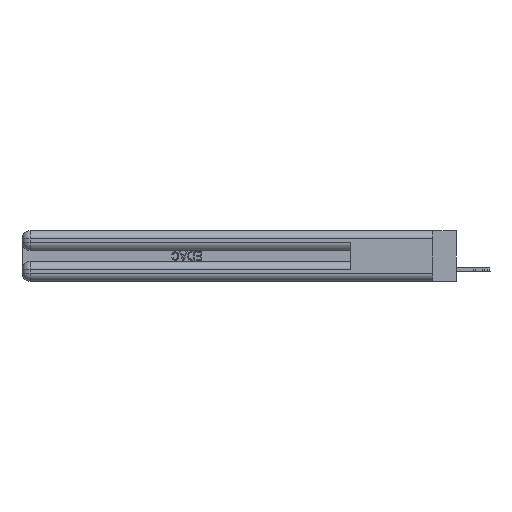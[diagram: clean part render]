
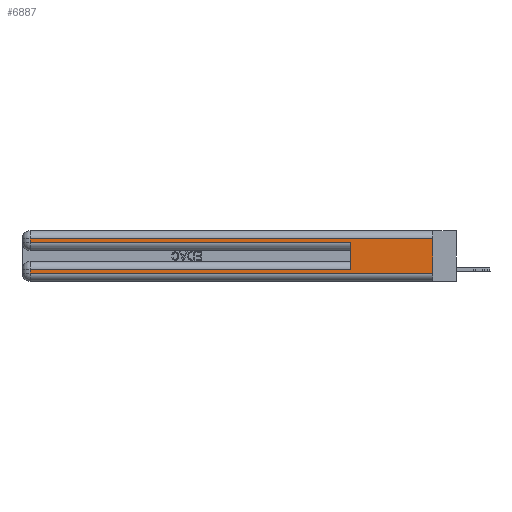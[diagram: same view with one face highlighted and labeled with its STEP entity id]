
A CAD part, left-side view. The second image highlights one B-rep face of the part: STEP entity #6887.
In plain terms, the highlighted planar face has unit normal (-1, 0, 0).
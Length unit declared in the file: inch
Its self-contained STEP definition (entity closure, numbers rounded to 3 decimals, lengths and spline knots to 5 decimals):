
#11 = CARTESIAN_POINT ( 'NONE',  ( 0., 0.6, 0.085 ) ) ;
#498 = VERTEX_POINT ( 'NONE', #2734 ) ;
#561 = LINE ( 'NONE', #31808, #43504 ) ;
#654 = VECTOR ( 'NONE', #34035, 39.37008 ) ;
#1411 = VERTEX_POINT ( 'NONE', #39035 ) ;
#1897 = CARTESIAN_POINT ( 'NONE',  ( 0., 0.6, 0.145 ) ) ;
#2085 = ORIENTED_EDGE ( 'NONE', *, *, #21250, .T. ) ;
#2146 = CARTESIAN_POINT ( 'NONE',  ( 0., 0., 0.06 ) ) ;
#2382 = EDGE_CURVE ( 'NONE', #1411, #4614, #21371, .T. ) ;
#2734 = CARTESIAN_POINT ( 'NONE',  ( 0., 0., 0.31 ) ) ;
#3222 = DIRECTION ( 'NONE',  ( 0., 0., -1. ) ) ;
#4614 = VERTEX_POINT ( 'NONE', #2146 ) ;
#5130 = CARTESIAN_POINT ( 'NONE',  ( 0., 0., 0.31 ) ) ;
#5215 = VERTEX_POINT ( 'NONE', #11 ) ;
#5454 = DIRECTION ( 'NONE',  ( 0., -1., 0. ) ) ;
#5567 = EDGE_CURVE ( 'NONE', #498, #4614, #10279, .T. ) ;
#5962 = CARTESIAN_POINT ( 'NONE',  ( 0., 0., 0.37 ) ) ;
#6195 = DIRECTION ( 'NONE',  ( 0., 0., -1. ) ) ;
#6257 = CARTESIAN_POINT ( 'NONE',  ( 0., 2.94, 0.31 ) ) ;
#6773 = ORIENTED_EDGE ( 'NONE', *, *, #25665, .T. ) ;
#6783 = VECTOR ( 'NONE', #5454, 39.37008 ) ;
#6887 = ADVANCED_FACE ( 'NONE', ( #19415 ), #13083, .F. ) ;
#7236 = CARTESIAN_POINT ( 'NONE',  ( 0., 2.94, 0.37 ) ) ;
#9448 = VECTOR ( 'NONE', #37033, 39.37008 ) ;
#9845 = VERTEX_POINT ( 'NONE', #15299 ) ;
#10125 = VERTEX_POINT ( 'NONE', #23908 ) ;
#10279 = LINE ( 'NONE', #17051, #654 ) ;
#10758 = ORIENTED_EDGE ( 'NONE', *, *, #46274, .T. ) ;
#12896 = CARTESIAN_POINT ( 'NONE',  ( 0., 0., 0.285 ) ) ;
#13076 = DIRECTION ( 'NONE',  ( 0., 0., 1. ) ) ;
#13083 = PLANE ( 'NONE',  #28054 ) ;
#13806 = ORIENTED_EDGE ( 'NONE', *, *, #2382, .T. ) ;
#15299 = CARTESIAN_POINT ( 'NONE',  ( 0., 2.94, 0.085 ) ) ;
#17051 = CARTESIAN_POINT ( 'NONE',  ( 0., 0., 0.37 ) ) ;
#17056 = DIRECTION ( 'NONE',  ( 0., 0., -1. ) ) ;
#17490 = DIRECTION ( 'NONE',  ( 0., 1., 0. ) ) ;
#18004 = ORIENTED_EDGE ( 'NONE', *, *, #33698, .F. ) ;
#19415 = FACE_OUTER_BOUND ( 'NONE', #30570, .T. ) ;
#19613 = VECTOR ( 'NONE', #13076, 39.37008 ) ;
#20991 = VECTOR ( 'NONE', #17490, 39.37008 ) ;
#21250 = EDGE_CURVE ( 'NONE', #5215, #9845, #46392, .T. ) ;
#21371 = LINE ( 'NONE', #37505, #9448 ) ;
#21771 = ORIENTED_EDGE ( 'NONE', *, *, #5567, .F. ) ;
#22453 = VECTOR ( 'NONE', #34040, 39.37008 ) ;
#23908 = CARTESIAN_POINT ( 'NONE',  ( 0., 2.94, 0.285 ) ) ;
#24373 = LINE ( 'NONE', #12896, #6783 ) ;
#25665 = EDGE_CURVE ( 'NONE', #30030, #10125, #561, .T. ) ;
#27537 = LINE ( 'NONE', #1897, #19613 ) ;
#28054 = AXIS2_PLACEMENT_3D ( 'NONE', #5962, #45623, #17056 ) ;
#29434 = VECTOR ( 'NONE', #3222, 39.37008 ) ;
#29924 = CARTESIAN_POINT ( 'NONE',  ( 0., 0.6, 0.285 ) ) ;
#30030 = VERTEX_POINT ( 'NONE', #6257 ) ;
#30570 = EDGE_LOOP ( 'NONE', ( #21771, #36864, #6773, #10758, #18004, #2085, #33802, #13806 ) ) ;
#31808 = CARTESIAN_POINT ( 'NONE',  ( 0., 2.94, 0.37 ) ) ;
#33698 = EDGE_CURVE ( 'NONE', #5215, #41396, #27537, .T. ) ;
#33802 = ORIENTED_EDGE ( 'NONE', *, *, #45904, .T. ) ;
#34035 = DIRECTION ( 'NONE',  ( 0., 0., -1. ) ) ;
#34040 = DIRECTION ( 'NONE',  ( 0., 1., 0. ) ) ;
#36864 = ORIENTED_EDGE ( 'NONE', *, *, #41401, .T. ) ;
#37033 = DIRECTION ( 'NONE',  ( 0., -1., 0. ) ) ;
#37505 = CARTESIAN_POINT ( 'NONE',  ( 0., 0., 0.06 ) ) ;
#38640 = CARTESIAN_POINT ( 'NONE',  ( 0., 0., 0.085 ) ) ;
#39035 = CARTESIAN_POINT ( 'NONE',  ( 0., 2.94, 0.06 ) ) ;
#40505 = LINE ( 'NONE', #5130, #22453 ) ;
#41396 = VERTEX_POINT ( 'NONE', #29924 ) ;
#41401 = EDGE_CURVE ( 'NONE', #498, #30030, #40505, .T. ) ;
#41862 = LINE ( 'NONE', #7236, #29434 ) ;
#43504 = VECTOR ( 'NONE', #6195, 39.37008 ) ;
#45623 = DIRECTION ( 'NONE',  ( 1., 0., 0. ) ) ;
#45904 = EDGE_CURVE ( 'NONE', #9845, #1411, #41862, .T. ) ;
#46274 = EDGE_CURVE ( 'NONE', #10125, #41396, #24373, .T. ) ;
#46392 = LINE ( 'NONE', #38640, #20991 ) ;
